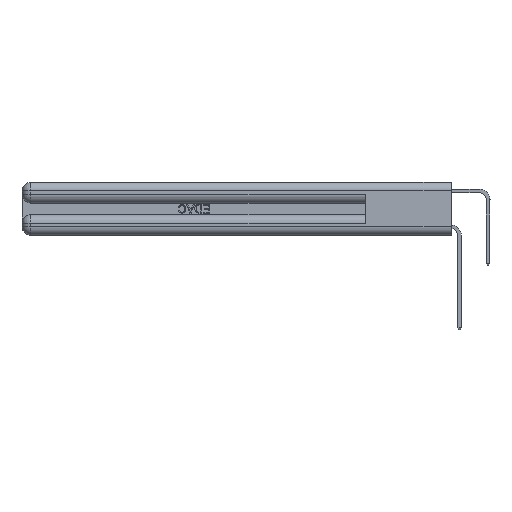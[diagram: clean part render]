
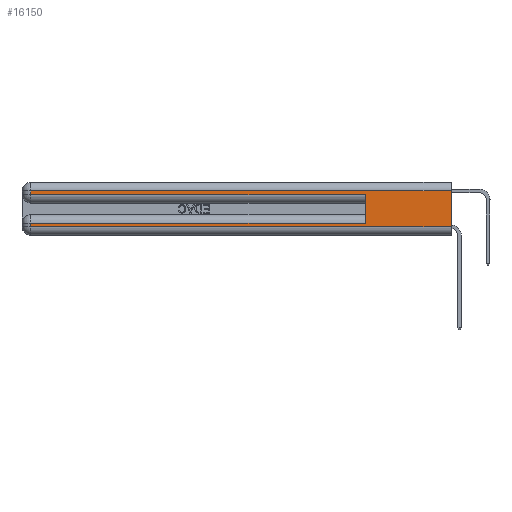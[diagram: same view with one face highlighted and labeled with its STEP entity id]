
A CAD part, left-side view. The second image highlights one B-rep face of the part: STEP entity #16150.
In plain terms, the highlighted planar face has unit normal (-1, 0, 0).
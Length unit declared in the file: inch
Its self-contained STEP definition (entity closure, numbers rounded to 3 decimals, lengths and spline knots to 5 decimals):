
#365 = CARTESIAN_POINT ( 'NONE',  ( 0., 2.94, 0.37 ) ) ;
#504 = CARTESIAN_POINT ( 'NONE',  ( 0., 2.94, 0.06 ) ) ;
#885 = DIRECTION ( 'NONE',  ( 0., 0., -1. ) ) ;
#989 = EDGE_CURVE ( 'NONE', #21450, #13896, #10319, .T. ) ;
#1982 = VECTOR ( 'NONE', #24957, 39.37008 ) ;
#2592 = CARTESIAN_POINT ( 'NONE',  ( 0., 0., 0.06 ) ) ;
#3022 = DIRECTION ( 'NONE',  ( 0., 0., -1. ) ) ;
#3068 = CARTESIAN_POINT ( 'NONE',  ( 0., 0.6, 0.285 ) ) ;
#3594 = LINE ( 'NONE', #13075, #10261 ) ;
#4286 = LINE ( 'NONE', #365, #32591 ) ;
#4440 = DIRECTION ( 'NONE',  ( 0., 0., -1. ) ) ;
#6206 = CARTESIAN_POINT ( 'NONE',  ( 0., 2.94, 0.285 ) ) ;
#6788 = VERTEX_POINT ( 'NONE', #504 ) ;
#6924 = CARTESIAN_POINT ( 'NONE',  ( 0., 2.94, 0.37 ) ) ;
#7173 = DIRECTION ( 'NONE',  ( 0., -1., 0. ) ) ;
#7992 = VECTOR ( 'NONE', #33552, 39.37008 ) ;
#8251 = LINE ( 'NONE', #25772, #25348 ) ;
#8619 = CARTESIAN_POINT ( 'NONE',  ( 0., 0., 0.085 ) ) ;
#9503 = EDGE_LOOP ( 'NONE', ( #10189, #24964, #10385, #11534, #12691, #13840, #27116, #17862 ) ) ;
#10090 = EDGE_CURVE ( 'NONE', #28771, #29335, #8251, .T. ) ;
#10189 = ORIENTED_EDGE ( 'NONE', *, *, #10090, .F. ) ;
#10261 = VECTOR ( 'NONE', #31681, 39.37008 ) ;
#10319 = LINE ( 'NONE', #17541, #26192 ) ;
#10385 = ORIENTED_EDGE ( 'NONE', *, *, #19278, .T. ) ;
#10416 = CARTESIAN_POINT ( 'NONE',  ( 0., 0., 0.37 ) ) ;
#11534 = ORIENTED_EDGE ( 'NONE', *, *, #989, .T. ) ;
#11707 = CARTESIAN_POINT ( 'NONE',  ( 0., 0., 0.31 ) ) ;
#11805 = DIRECTION ( 'NONE',  ( 0., -1., 0. ) ) ;
#12691 = ORIENTED_EDGE ( 'NONE', *, *, #22388, .F. ) ;
#13075 = CARTESIAN_POINT ( 'NONE',  ( 0., 0.6, 0.145 ) ) ;
#13840 = ORIENTED_EDGE ( 'NONE', *, *, #21299, .T. ) ;
#13896 = VERTEX_POINT ( 'NONE', #3068 ) ;
#16150 = ADVANCED_FACE ( 'NONE', ( #19441 ), #34000, .F. ) ;
#16333 = LINE ( 'NONE', #6924, #7992 ) ;
#16515 = VECTOR ( 'NONE', #28330, 39.37008 ) ;
#17541 = CARTESIAN_POINT ( 'NONE',  ( 0., 0., 0.285 ) ) ;
#17862 = ORIENTED_EDGE ( 'NONE', *, *, #23980, .T. ) ;
#19268 = CARTESIAN_POINT ( 'NONE',  ( 0., 2.94, 0.31 ) ) ;
#19278 = EDGE_CURVE ( 'NONE', #26206, #21450, #16333, .T. ) ;
#19441 = FACE_OUTER_BOUND ( 'NONE', #9503, .T. ) ;
#19833 = LINE ( 'NONE', #11707, #16515 ) ;
#19894 = LINE ( 'NONE', #8619, #1982 ) ;
#20201 = LINE ( 'NONE', #21979, #32684 ) ;
#20627 = CARTESIAN_POINT ( 'NONE',  ( 0., 2.94, 0.085 ) ) ;
#21299 = EDGE_CURVE ( 'NONE', #21459, #31235, #19894, .T. ) ;
#21450 = VERTEX_POINT ( 'NONE', #6206 ) ;
#21459 = VERTEX_POINT ( 'NONE', #25431 ) ;
#21979 = CARTESIAN_POINT ( 'NONE',  ( 0., 0., 0.06 ) ) ;
#22388 = EDGE_CURVE ( 'NONE', #21459, #13896, #3594, .T. ) ;
#23366 = EDGE_CURVE ( 'NONE', #28771, #26206, #19833, .T. ) ;
#23980 = EDGE_CURVE ( 'NONE', #6788, #29335, #20201, .T. ) ;
#24957 = DIRECTION ( 'NONE',  ( 0., 1., 0. ) ) ;
#24964 = ORIENTED_EDGE ( 'NONE', *, *, #23366, .T. ) ;
#25348 = VECTOR ( 'NONE', #4440, 39.37008 ) ;
#25431 = CARTESIAN_POINT ( 'NONE',  ( 0., 0.6, 0.085 ) ) ;
#25772 = CARTESIAN_POINT ( 'NONE',  ( 0., 0., 0.37 ) ) ;
#26192 = VECTOR ( 'NONE', #7173, 39.37008 ) ;
#26206 = VERTEX_POINT ( 'NONE', #19268 ) ;
#26641 = AXIS2_PLACEMENT_3D ( 'NONE', #10416, #32372, #885 ) ;
#26975 = CARTESIAN_POINT ( 'NONE',  ( 0., 0., 0.31 ) ) ;
#27116 = ORIENTED_EDGE ( 'NONE', *, *, #29867, .T. ) ;
#28330 = DIRECTION ( 'NONE',  ( 0., 1., 0. ) ) ;
#28771 = VERTEX_POINT ( 'NONE', #26975 ) ;
#29335 = VERTEX_POINT ( 'NONE', #2592 ) ;
#29867 = EDGE_CURVE ( 'NONE', #31235, #6788, #4286, .T. ) ;
#31235 = VERTEX_POINT ( 'NONE', #20627 ) ;
#31681 = DIRECTION ( 'NONE',  ( 0., 0., 1. ) ) ;
#32372 = DIRECTION ( 'NONE',  ( 1., 0., 0. ) ) ;
#32591 = VECTOR ( 'NONE', #3022, 39.37008 ) ;
#32684 = VECTOR ( 'NONE', #11805, 39.37008 ) ;
#33552 = DIRECTION ( 'NONE',  ( 0., 0., -1. ) ) ;
#34000 = PLANE ( 'NONE',  #26641 ) ;
